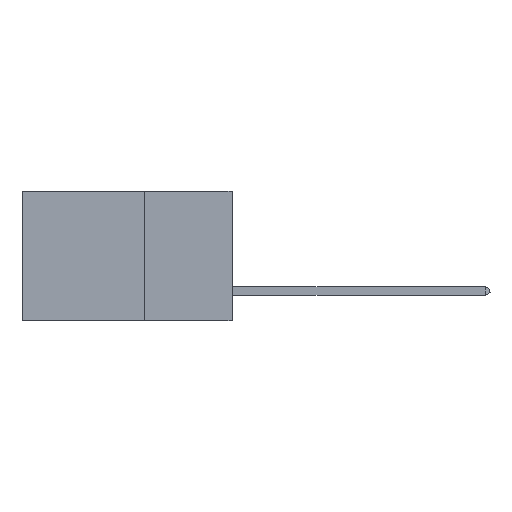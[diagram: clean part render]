
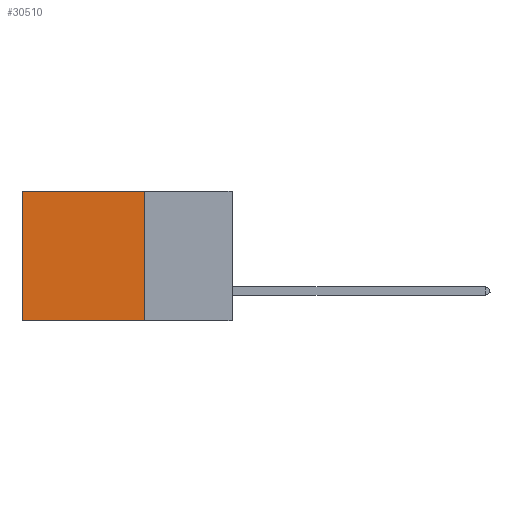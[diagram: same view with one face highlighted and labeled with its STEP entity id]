
A CAD part, left-side view. The second image highlights one B-rep face of the part: STEP entity #30510.
In plain terms, the highlighted planar face has unit normal (-1, 0, 0).
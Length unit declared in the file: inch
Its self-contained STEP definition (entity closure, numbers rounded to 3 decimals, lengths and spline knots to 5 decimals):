
#3566 = VERTEX_POINT ( 'NONE', #15004 ) ;
#5675 = EDGE_LOOP ( 'NONE', ( #26356, #20071, #21891, #12044 ) ) ;
#6159 = EDGE_CURVE ( 'NONE', #3566, #9928, #21758, .T. ) ;
#6628 = DIRECTION ( 'NONE',  ( 0., 1., 0. ) ) ;
#6634 = VECTOR ( 'NONE', #29320, 39.37008 ) ;
#6715 = EDGE_CURVE ( 'NONE', #3566, #8232, #25660, .T. ) ;
#7001 = DIRECTION ( 'NONE',  ( 0., 0., -1. ) ) ;
#7433 = EDGE_CURVE ( 'NONE', #8232, #7705, #11181, .T. ) ;
#7705 = VERTEX_POINT ( 'NONE', #28950 ) ;
#8232 = VERTEX_POINT ( 'NONE', #9632 ) ;
#9337 = EDGE_CURVE ( 'NONE', #9928, #7705, #19624, .T. ) ;
#9632 = CARTESIAN_POINT ( 'NONE',  ( 0.2875, 0.25, -0.37 ) ) ;
#9928 = VERTEX_POINT ( 'NONE', #29099 ) ;
#10783 = AXIS2_PLACEMENT_3D ( 'NONE', #28576, #14336, #7001 ) ;
#11181 = LINE ( 'NONE', #13875, #17865 ) ;
#12044 = ORIENTED_EDGE ( 'NONE', *, *, #6159, .T. ) ;
#13875 = CARTESIAN_POINT ( 'NONE',  ( 0.2875, 0.25, -0.37 ) ) ;
#14336 = DIRECTION ( 'NONE',  ( 1., 0., 0. ) ) ;
#14571 = CARTESIAN_POINT ( 'NONE',  ( 0.2875, 0.6, 0. ) ) ;
#15004 = CARTESIAN_POINT ( 'NONE',  ( 0.2875, 0.25, 0. ) ) ;
#15507 = DIRECTION ( 'NONE',  ( 0., 1., 0. ) ) ;
#17865 = VECTOR ( 'NONE', #6628, 39.37008 ) ;
#19624 = LINE ( 'NONE', #14571, #21109 ) ;
#20071 = ORIENTED_EDGE ( 'NONE', *, *, #7433, .F. ) ;
#20279 = VECTOR ( 'NONE', #15507, 39.37008 ) ;
#21109 = VECTOR ( 'NONE', #21824, 39.37008 ) ;
#21758 = LINE ( 'NONE', #22441, #20279 ) ;
#21824 = DIRECTION ( 'NONE',  ( 0., 0., -1. ) ) ;
#21891 = ORIENTED_EDGE ( 'NONE', *, *, #6715, .F. ) ;
#22441 = CARTESIAN_POINT ( 'NONE',  ( 0.2875, 0.25, 0. ) ) ;
#23983 = PLANE ( 'NONE',  #10783 ) ;
#25660 = LINE ( 'NONE', #29212, #6634 ) ;
#26356 = ORIENTED_EDGE ( 'NONE', *, *, #9337, .T. ) ;
#28576 = CARTESIAN_POINT ( 'NONE',  ( 0.2875, 0.25, 0. ) ) ;
#28950 = CARTESIAN_POINT ( 'NONE',  ( 0.2875, 0.6, -0.37 ) ) ;
#29099 = CARTESIAN_POINT ( 'NONE',  ( 0.2875, 0.6, 0. ) ) ;
#29212 = CARTESIAN_POINT ( 'NONE',  ( 0.2875, 0.25, 0. ) ) ;
#29320 = DIRECTION ( 'NONE',  ( 0., 0., -1. ) ) ;
#29352 = FACE_OUTER_BOUND ( 'NONE', #5675, .T. ) ;
#30510 = ADVANCED_FACE ( 'NONE', ( #29352 ), #23983, .F. ) ;
